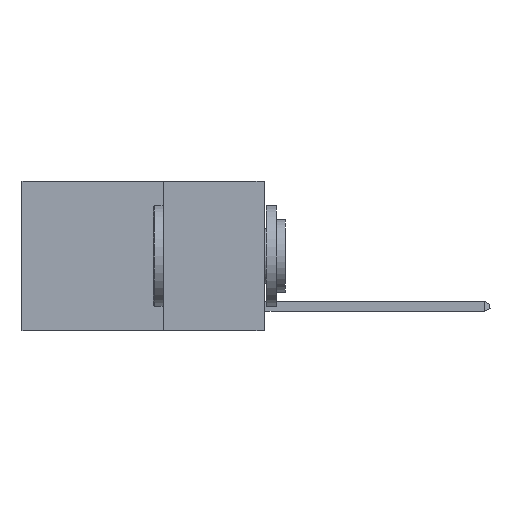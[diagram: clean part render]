
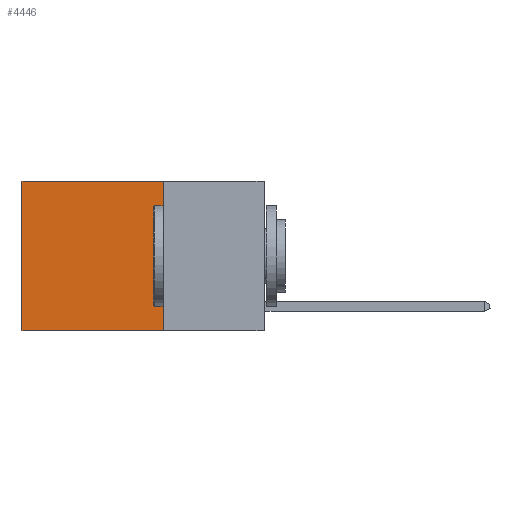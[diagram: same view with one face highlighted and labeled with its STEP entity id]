
A CAD part, left-side view. The second image highlights one B-rep face of the part: STEP entity #4446.
In plain terms, the highlighted planar face has unit normal (-1, 0, 0).
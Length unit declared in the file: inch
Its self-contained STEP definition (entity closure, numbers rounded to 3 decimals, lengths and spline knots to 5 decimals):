
#136 = CARTESIAN_POINT ( 'NONE',  ( 0.2625, 0.6, 0. ) ) ;
#280 = LINE ( 'NONE', #3397, #3316 ) ;
#753 = LINE ( 'NONE', #7021, #1271 ) ;
#1271 = VECTOR ( 'NONE', #4172, 39.37008 ) ;
#1322 = CARTESIAN_POINT ( 'NONE',  ( 0.2625, 0.6, -0.37 ) ) ;
#1380 = PLANE ( 'NONE',  #8504 ) ;
#1733 = CARTESIAN_POINT ( 'NONE',  ( 0.2625, 0.25, -0.37 ) ) ;
#1803 = ORIENTED_EDGE ( 'NONE', *, *, #9120, .T. ) ;
#1946 = LINE ( 'NONE', #8042, #1996 ) ;
#1947 = DIRECTION ( 'NONE',  ( 1., 0., 0. ) ) ;
#1996 = VECTOR ( 'NONE', #8805, 39.37008 ) ;
#1998 = FACE_OUTER_BOUND ( 'NONE', #7886, .T. ) ;
#2426 = VECTOR ( 'NONE', #4685, 39.37008 ) ;
#3316 = VECTOR ( 'NONE', #6523, 39.37008 ) ;
#3397 = CARTESIAN_POINT ( 'NONE',  ( 0.2625, 0.25, -0.37 ) ) ;
#3994 = EDGE_CURVE ( 'NONE', #9457, #9287, #5587, .T. ) ;
#4172 = DIRECTION ( 'NONE',  ( 0., 0., -1. ) ) ;
#4446 = ADVANCED_FACE ( 'NONE', ( #1998 ), #1380, .F. ) ;
#4685 = DIRECTION ( 'NONE',  ( 0., 0., -1. ) ) ;
#5140 = DIRECTION ( 'NONE',  ( 0., 0., -1. ) ) ;
#5587 = LINE ( 'NONE', #136, #2426 ) ;
#5959 = EDGE_CURVE ( 'NONE', #7117, #8580, #753, .T. ) ;
#6243 = CARTESIAN_POINT ( 'NONE',  ( 0.2625, 0.25, 0. ) ) ;
#6523 = DIRECTION ( 'NONE',  ( 0., 1., 0. ) ) ;
#7021 = CARTESIAN_POINT ( 'NONE',  ( 0.2625, 0.25, 0. ) ) ;
#7117 = VERTEX_POINT ( 'NONE', #6243 ) ;
#7334 = ORIENTED_EDGE ( 'NONE', *, *, #9184, .F. ) ;
#7886 = EDGE_LOOP ( 'NONE', ( #9440, #7334, #8206, #1803 ) ) ;
#8042 = CARTESIAN_POINT ( 'NONE',  ( 0.2625, 0.25, 0. ) ) ;
#8206 = ORIENTED_EDGE ( 'NONE', *, *, #5959, .F. ) ;
#8504 = AXIS2_PLACEMENT_3D ( 'NONE', #9199, #1947, #5140 ) ;
#8580 = VERTEX_POINT ( 'NONE', #1733 ) ;
#8805 = DIRECTION ( 'NONE',  ( 0., 1., 0. ) ) ;
#9120 = EDGE_CURVE ( 'NONE', #7117, #9457, #1946, .T. ) ;
#9184 = EDGE_CURVE ( 'NONE', #8580, #9287, #280, .T. ) ;
#9199 = CARTESIAN_POINT ( 'NONE',  ( 0.2625, 0.25, 0. ) ) ;
#9287 = VERTEX_POINT ( 'NONE', #1322 ) ;
#9403 = CARTESIAN_POINT ( 'NONE',  ( 0.2625, 0.6, 0. ) ) ;
#9440 = ORIENTED_EDGE ( 'NONE', *, *, #3994, .T. ) ;
#9457 = VERTEX_POINT ( 'NONE', #9403 ) ;
